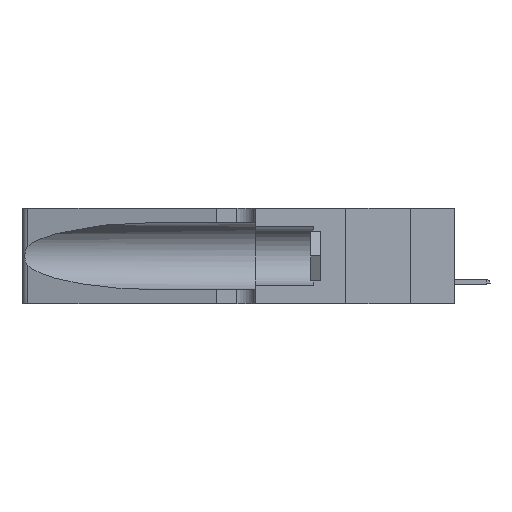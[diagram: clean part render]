
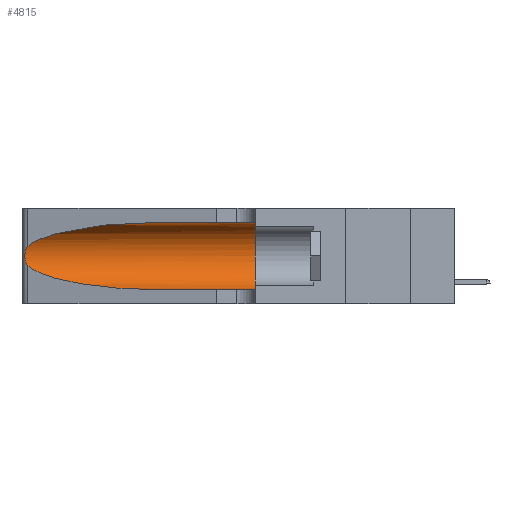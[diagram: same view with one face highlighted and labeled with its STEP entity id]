
A CAD part, left-side view. The second image highlights one B-rep face of the part: STEP entity #4815.
In plain terms, the highlighted cylindrical face has radius 3.308 mm (diameter 6.617 mm), a partial arc.
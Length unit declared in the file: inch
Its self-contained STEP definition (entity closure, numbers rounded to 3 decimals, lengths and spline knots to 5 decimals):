
#1306 = CYLINDRICAL_SURFACE ( 'NONE', #19094, 0.13025 ) ;
#1556 =( BOUNDED_CURVE ( )  B_SPLINE_CURVE ( 3, ( #11113, #23351, #17727, #8505 ),
 .UNSPECIFIED., .F., .F. ) 
 B_SPLINE_CURVE_WITH_KNOTS ( ( 4, 4 ),
 ( 1.5708, 2.84003 ),
 .UNSPECIFIED. ) 
 CURVE ( )  GEOMETRIC_REPRESENTATION_ITEM ( )  RATIONAL_B_SPLINE_CURVE ( ( 1., 0.87, 0.87, 1. ) ) 
 REPRESENTATION_ITEM ( '' )  );
#2752 = ORIENTED_EDGE ( 'NONE', *, *, #3697, .T. ) ;
#3407 = DIRECTION ( 'NONE',  ( 0., 1., 0. ) ) ;
#3570 = CARTESIAN_POINT ( 'NONE',  ( 0.1305, 1.61858, 0.185 ) ) ;
#3697 = EDGE_CURVE ( 'NONE', #27955, #27829, #16678, .T. ) ;
#4494 = VERTEX_POINT ( 'NONE', #37048 ) ;
#4624 = CARTESIAN_POINT ( 'NONE',  ( 0.25487, 1.22718, 0.22369 ) ) ;
#4815 = ADVANCED_FACE ( 'NONE', ( #30839 ), #1306, .F. ) ;
#5051 = LINE ( 'NONE', #17884, #20916 ) ;
#5203 = EDGE_CURVE ( 'NONE', #10737, #27955, #28531, .T. ) ;
#5341 = CARTESIAN_POINT ( 'NONE',  ( 0.25487, 1.22718, 0.22369 ) ) ;
#6418 = DIRECTION ( 'NONE',  ( 0., 0., 1. ) ) ;
#6469 = CARTESIAN_POINT ( 'NONE',  ( 0.1305, 0.72297, 0.05475 ) ) ;
#8144 = CARTESIAN_POINT ( 'NONE',  ( 0.26017, 1.23833, 0.17102 ) ) ;
#8259 = DIRECTION ( 'NONE',  ( 0., -1., 0. ) ) ;
#8505 = CARTESIAN_POINT ( 'NONE',  ( 0.25487, 1.22718, 0.22369 ) ) ;
#9169 = VERTEX_POINT ( 'NONE', #26506 ) ;
#9220 = CIRCLE ( 'NONE', #22015, 0.13025 ) ;
#9397 = DIRECTION ( 'NONE',  ( 0., 0., -1. ) ) ;
#9423 = ORIENTED_EDGE ( 'NONE', *, *, #36776, .F. ) ;
#10737 = VERTEX_POINT ( 'NONE', #4624 ) ;
#11113 = CARTESIAN_POINT ( 'NONE',  ( 0.1305, 0.72297, 0.31525 ) ) ;
#11157 = CARTESIAN_POINT ( 'NONE',  ( 0.25639, 1.23184, 0.21858 ) ) ;
#11347 = CARTESIAN_POINT ( 'NONE',  ( 0.25487, 1.22718, 0.14631 ) ) ;
#11547 = CARTESIAN_POINT ( 'NONE',  ( 0.25639, 1.23186, 0.15144 ) ) ;
#11674 = CARTESIAN_POINT ( 'NONE',  ( 0.25487, 1.22718, 0.14631 ) ) ;
#12430 = ORIENTED_EDGE ( 'NONE', *, *, #25375, .T. ) ;
#12670 = CARTESIAN_POINT ( 'NONE',  ( 0.25487, 1.22718, 0.14631 ) ) ;
#12744 = EDGE_LOOP ( 'NONE', ( #39340, #14890, #2752, #12430, #9423, #38984 ) ) ;
#13268 = CARTESIAN_POINT ( 'NONE',  ( 0.2373, 1.15595, 0.08982 ) ) ;
#14890 = ORIENTED_EDGE ( 'NONE', *, *, #5203, .T. ) ;
#16678 =( BOUNDED_CURVE ( )  B_SPLINE_CURVE ( 3, ( #12670, #13268, #22107, #6469 ),
 .UNSPECIFIED., .F., .F. ) 
 B_SPLINE_CURVE_WITH_KNOTS ( ( 4, 4 ),
 ( 3.44316, 4.71239 ),
 .UNSPECIFIED. ) 
 CURVE ( )  GEOMETRIC_REPRESENTATION_ITEM ( )  RATIONAL_B_SPLINE_CURVE ( ( 1., 0.87, 0.87, 1. ) ) 
 REPRESENTATION_ITEM ( '' )  );
#16997 = CARTESIAN_POINT ( 'NONE',  ( 0.25787, 1.23484, 0.2124 ) ) ;
#17727 = CARTESIAN_POINT ( 'NONE',  ( 0.2373, 1.15595, 0.28018 ) ) ;
#17884 = CARTESIAN_POINT ( 'NONE',  ( 0.1305, 1.61858, 0.05475 ) ) ;
#17900 = CARTESIAN_POINT ( 'NONE',  ( 0.1305, 0.72297, 0.05475 ) ) ;
#19094 = AXIS2_PLACEMENT_3D ( 'NONE', #3570, #37001, #9397 ) ;
#19311 = LINE ( 'NONE', #28515, #24875 ) ;
#20286 = CARTESIAN_POINT ( 'NONE',  ( 0.1305, 0.35, 0.05475 ) ) ;
#20580 = CARTESIAN_POINT ( 'NONE',  ( 0.25555, 1.22994, 0.2215 ) ) ;
#20777 = CARTESIAN_POINT ( 'NONE',  ( 0.26075, 1.23896, 0.19203 ) ) ;
#20916 = VECTOR ( 'NONE', #8259, 39.37008 ) ;
#22015 = AXIS2_PLACEMENT_3D ( 'NONE', #27479, #3407, #6418 ) ;
#22107 = CARTESIAN_POINT ( 'NONE',  ( 0.18966, 0.96281, 0.05475 ) ) ;
#22109 = DIRECTION ( 'NONE',  ( 0., -1., 0. ) ) ;
#23351 = CARTESIAN_POINT ( 'NONE',  ( 0.18966, 0.96281, 0.31525 ) ) ;
#24875 = VECTOR ( 'NONE', #22109, 39.37008 ) ;
#24912 = EDGE_CURVE ( 'NONE', #9169, #10737, #1556, .T. ) ;
#25375 = EDGE_CURVE ( 'NONE', #27829, #25489, #5051, .T. ) ;
#25489 = VERTEX_POINT ( 'NONE', #20286 ) ;
#26506 = CARTESIAN_POINT ( 'NONE',  ( 0.1305, 0.72297, 0.31525 ) ) ;
#26594 = CARTESIAN_POINT ( 'NONE',  ( 0.25789, 1.23486, 0.15765 ) ) ;
#26787 = CARTESIAN_POINT ( 'NONE',  ( 0.25856, 1.23593, 0.16098 ) ) ;
#27479 = CARTESIAN_POINT ( 'NONE',  ( 0.1305, 0.35, 0.185 ) ) ;
#27829 = VERTEX_POINT ( 'NONE', #17900 ) ;
#27955 = VERTEX_POINT ( 'NONE', #11674 ) ;
#28515 = CARTESIAN_POINT ( 'NONE',  ( 0.1305, 1.61858, 0.31525 ) ) ;
#28531 = B_SPLINE_CURVE_WITH_KNOTS ( 'NONE', 3,
 ( #5341, #20580, #11157, #16997, #32576, #29780, #20777, #29400, #8144, #26787, #26594, #11547, #38760, #11347 ),
 .UNSPECIFIED., .F., .F.,
 ( 4, 2, 2, 2, 2, 2, 4 ),
 ( 0., 0.00027, 0.00053, 0.00107, 0.0016, 0.00187, 0.00214 ),
 .UNSPECIFIED. ) ;
#29400 = CARTESIAN_POINT ( 'NONE',  ( 0.26075, 1.23896, 0.178 ) ) ;
#29780 = CARTESIAN_POINT ( 'NONE',  ( 0.26018, 1.23835, 0.19895 ) ) ;
#30839 = FACE_OUTER_BOUND ( 'NONE', #12744, .T. ) ;
#32576 = CARTESIAN_POINT ( 'NONE',  ( 0.25854, 1.2359, 0.20912 ) ) ;
#36776 = EDGE_CURVE ( 'NONE', #4494, #25489, #9220, .T. ) ;
#37001 = DIRECTION ( 'NONE',  ( 0., -1., 0. ) ) ;
#37048 = CARTESIAN_POINT ( 'NONE',  ( 0.1305, 0.35, 0.31525 ) ) ;
#37760 = EDGE_CURVE ( 'NONE', #9169, #4494, #19311, .T. ) ;
#38760 = CARTESIAN_POINT ( 'NONE',  ( 0.25555, 1.22993, 0.14849 ) ) ;
#38984 = ORIENTED_EDGE ( 'NONE', *, *, #37760, .F. ) ;
#39340 = ORIENTED_EDGE ( 'NONE', *, *, #24912, .T. ) ;
